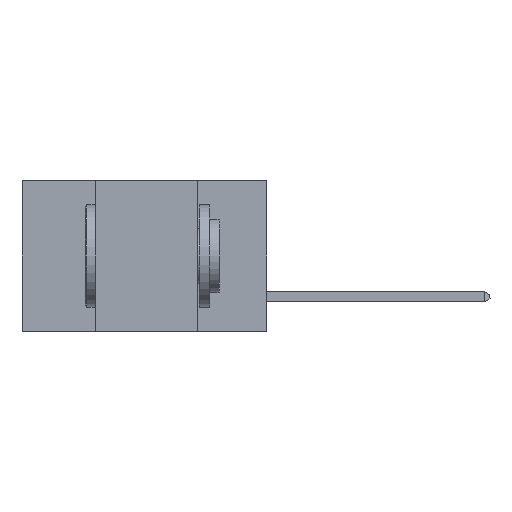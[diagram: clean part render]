
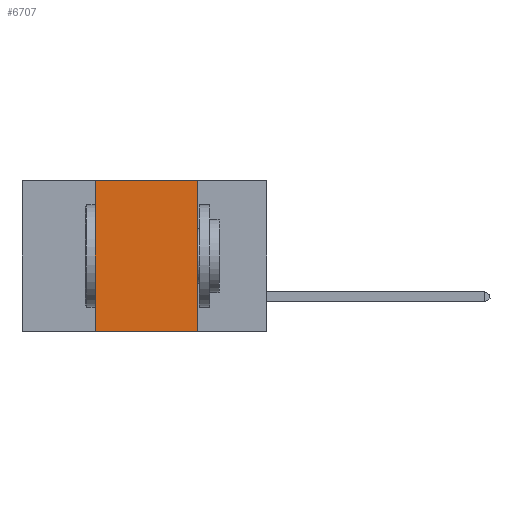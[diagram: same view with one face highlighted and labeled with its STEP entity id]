
A CAD part, left-side view. The second image highlights one B-rep face of the part: STEP entity #6707.
In plain terms, the highlighted planar face has unit normal (-1, 0, 0).
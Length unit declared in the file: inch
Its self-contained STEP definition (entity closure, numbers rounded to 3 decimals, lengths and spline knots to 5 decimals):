
#113 = LINE ( 'NONE', #5050, #3734 ) ;
#191 = DIRECTION ( 'NONE',  ( 1., 0., 0. ) ) ;
#220 = VECTOR ( 'NONE', #13026, 39.37008 ) ;
#364 = CARTESIAN_POINT ( 'NONE',  ( 0., 0.42, -0.37 ) ) ;
#2170 = CARTESIAN_POINT ( 'NONE',  ( 0., 0.6, 0. ) ) ;
#2330 = CARTESIAN_POINT ( 'NONE',  ( 0., 0.42, 0. ) ) ;
#2357 = CARTESIAN_POINT ( 'NONE',  ( 0., 0.42, 0. ) ) ;
#2380 = VECTOR ( 'NONE', #9393, 39.37008 ) ;
#2460 = VECTOR ( 'NONE', #5956, 39.37008 ) ;
#2558 = EDGE_CURVE ( 'NONE', #9428, #4802, #9315, .T. ) ;
#2667 = CARTESIAN_POINT ( 'NONE',  ( 0., 0.17, 0. ) ) ;
#3734 = VECTOR ( 'NONE', #13483, 39.37008 ) ;
#4050 = LINE ( 'NONE', #2170, #220 ) ;
#4663 = EDGE_CURVE ( 'NONE', #4802, #14587, #4050, .T. ) ;
#4802 = VERTEX_POINT ( 'NONE', #2330 ) ;
#5050 = CARTESIAN_POINT ( 'NONE',  ( 0., 0.6, -0.37 ) ) ;
#5956 = DIRECTION ( 'NONE',  ( 0., 0., 1. ) ) ;
#6224 = PLANE ( 'NONE',  #15617 ) ;
#6279 = CARTESIAN_POINT ( 'NONE',  ( 0., 0.6, 0. ) ) ;
#6707 = ADVANCED_FACE ( 'NONE', ( #11586 ), #6224, .F. ) ;
#9315 = LINE ( 'NONE', #2357, #2460 ) ;
#9393 = DIRECTION ( 'NONE',  ( 0., 0., -1. ) ) ;
#9428 = VERTEX_POINT ( 'NONE', #364 ) ;
#9641 = ORIENTED_EDGE ( 'NONE', *, *, #13763, .F. ) ;
#9932 = DIRECTION ( 'NONE',  ( 0., 0., -1. ) ) ;
#10092 = ORIENTED_EDGE ( 'NONE', *, *, #4663, .F. ) ;
#10314 = VERTEX_POINT ( 'NONE', #13445 ) ;
#11586 = FACE_OUTER_BOUND ( 'NONE', #14896, .T. ) ;
#13026 = DIRECTION ( 'NONE',  ( 0., -1., 0. ) ) ;
#13066 = CARTESIAN_POINT ( 'NONE',  ( 0., 0.17, 0. ) ) ;
#13445 = CARTESIAN_POINT ( 'NONE',  ( 0., 0.17, -0.37 ) ) ;
#13483 = DIRECTION ( 'NONE',  ( 0., -1., 0. ) ) ;
#13600 = LINE ( 'NONE', #13066, #2380 ) ;
#13763 = EDGE_CURVE ( 'NONE', #14587, #10314, #13600, .T. ) ;
#13879 = ORIENTED_EDGE ( 'NONE', *, *, #2558, .F. ) ;
#13889 = EDGE_CURVE ( 'NONE', #9428, #10314, #113, .T. ) ;
#13923 = ORIENTED_EDGE ( 'NONE', *, *, #13889, .T. ) ;
#14587 = VERTEX_POINT ( 'NONE', #2667 ) ;
#14896 = EDGE_LOOP ( 'NONE', ( #9641, #10092, #13879, #13923 ) ) ;
#15617 = AXIS2_PLACEMENT_3D ( 'NONE', #6279, #191, #9932 ) ;
